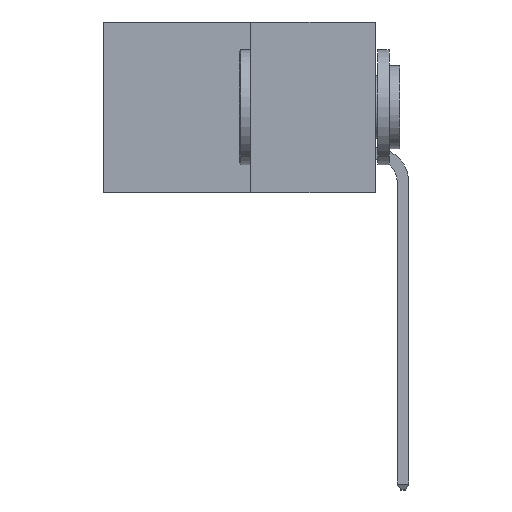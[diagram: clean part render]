
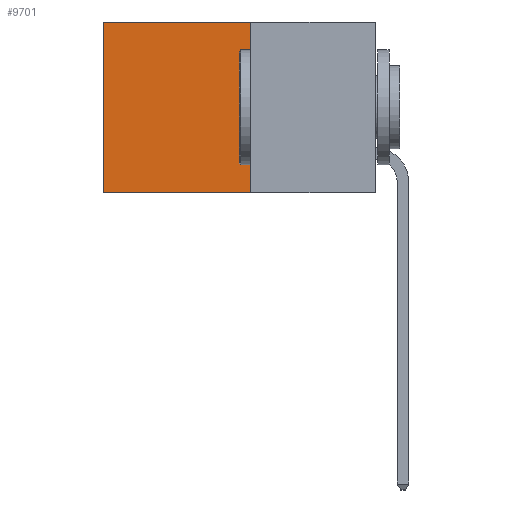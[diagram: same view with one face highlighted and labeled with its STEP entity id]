
A CAD part, left-side view. The second image highlights one B-rep face of the part: STEP entity #9701.
In plain terms, the highlighted planar face has unit normal (-1, 0, 0).
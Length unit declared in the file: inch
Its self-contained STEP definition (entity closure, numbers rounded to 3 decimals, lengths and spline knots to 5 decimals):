
#1679 = AXIS2_PLACEMENT_3D ( 'NONE', #3106, #4631, #10024 ) ;
#2000 = FACE_OUTER_BOUND ( 'NONE', #8047, .T. ) ;
#2112 = CARTESIAN_POINT ( 'NONE',  ( 0.277, 0.27, -0.37 ) ) ;
#2242 = PLANE ( 'NONE',  #1679 ) ;
#2677 = VERTEX_POINT ( 'NONE', #8758 ) ;
#3019 = LINE ( 'NONE', #2112, #7124 ) ;
#3101 = EDGE_CURVE ( 'NONE', #2677, #8128, #3019, .T. ) ;
#3106 = CARTESIAN_POINT ( 'NONE',  ( 0.277, 0.27, -0.37 ) ) ;
#3120 = LINE ( 'NONE', #4272, #9037 ) ;
#3164 = CARTESIAN_POINT ( 'NONE',  ( 0.277, 0.59, -0.37 ) ) ;
#3455 = LINE ( 'NONE', #6062, #7316 ) ;
#4110 = EDGE_CURVE ( 'NONE', #5253, #7294, #3120, .T. ) ;
#4272 = CARTESIAN_POINT ( 'NONE',  ( 0.277, 0.59, -0.37 ) ) ;
#4631 = DIRECTION ( 'NONE',  ( 1., 0., 0. ) ) ;
#5144 = DIRECTION ( 'NONE',  ( 0., 1., 0. ) ) ;
#5253 = VERTEX_POINT ( 'NONE', #7243 ) ;
#5443 = EDGE_CURVE ( 'NONE', #8128, #7294, #3455, .T. ) ;
#5609 = CARTESIAN_POINT ( 'NONE',  ( 0.277, 0.27, -0.37 ) ) ;
#5758 = ORIENTED_EDGE ( 'NONE', *, *, #6424, .T. ) ;
#5939 = DIRECTION ( 'NONE',  ( 0., 1., 0. ) ) ;
#5977 = VECTOR ( 'NONE', #5144, 39.37008 ) ;
#6062 = CARTESIAN_POINT ( 'NONE',  ( 0.277, 0.27, -0.37 ) ) ;
#6147 = DIRECTION ( 'NONE',  ( 0., 0., -1. ) ) ;
#6265 = CARTESIAN_POINT ( 'NONE',  ( 0.277, 0.27, 0. ) ) ;
#6424 = EDGE_CURVE ( 'NONE', #2677, #5253, #10092, .T. ) ;
#7124 = VECTOR ( 'NONE', #6147, 39.37008 ) ;
#7140 = ORIENTED_EDGE ( 'NONE', *, *, #4110, .T. ) ;
#7243 = CARTESIAN_POINT ( 'NONE',  ( 0.277, 0.59, 0. ) ) ;
#7294 = VERTEX_POINT ( 'NONE', #3164 ) ;
#7316 = VECTOR ( 'NONE', #5939, 39.37008 ) ;
#8047 = EDGE_LOOP ( 'NONE', ( #7140, #9057, #9985, #5758 ) ) ;
#8128 = VERTEX_POINT ( 'NONE', #5609 ) ;
#8758 = CARTESIAN_POINT ( 'NONE',  ( 0.277, 0.27, 0. ) ) ;
#9037 = VECTOR ( 'NONE', #9386, 39.37008 ) ;
#9057 = ORIENTED_EDGE ( 'NONE', *, *, #5443, .F. ) ;
#9386 = DIRECTION ( 'NONE',  ( 0., 0., -1. ) ) ;
#9701 = ADVANCED_FACE ( 'NONE', ( #2000 ), #2242, .F. ) ;
#9985 = ORIENTED_EDGE ( 'NONE', *, *, #3101, .F. ) ;
#10024 = DIRECTION ( 'NONE',  ( 0., 0., -1. ) ) ;
#10092 = LINE ( 'NONE', #6265, #5977 ) ;
